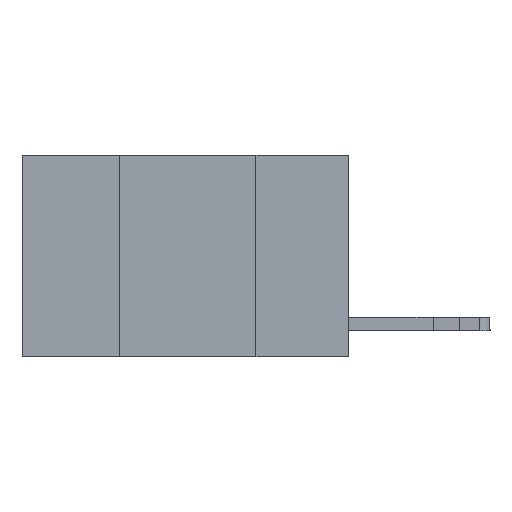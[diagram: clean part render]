
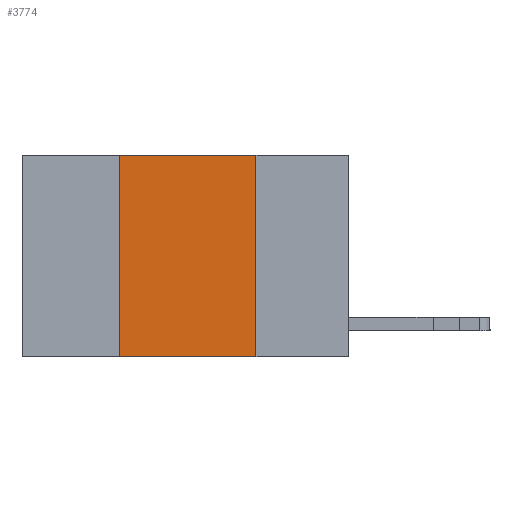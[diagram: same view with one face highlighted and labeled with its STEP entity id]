
A CAD part, left-side view. The second image highlights one B-rep face of the part: STEP entity #3774.
In plain terms, the highlighted planar face has unit normal (-1, 0, 0).
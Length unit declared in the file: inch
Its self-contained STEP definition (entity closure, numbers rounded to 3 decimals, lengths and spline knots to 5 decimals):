
#254 = EDGE_LOOP ( 'NONE', ( #4907, #4787, #3917, #13161 ) ) ;
#516 = LINE ( 'NONE', #7044, #6135 ) ;
#1281 = DIRECTION ( 'NONE',  ( 0., -1., 0. ) ) ;
#1306 = EDGE_CURVE ( 'NONE', #3032, #5021, #10308, .T. ) ;
#1442 = LINE ( 'NONE', #4758, #10505 ) ;
#1938 = AXIS2_PLACEMENT_3D ( 'NONE', #4579, #7053, #9041 ) ;
#2400 = LINE ( 'NONE', #3845, #10795 ) ;
#2567 = EDGE_CURVE ( 'NONE', #10927, #14480, #1442, .T. ) ;
#2594 = CARTESIAN_POINT ( 'NONE',  ( 0., 0.42, -0.37 ) ) ;
#2740 = DIRECTION ( 'NONE',  ( 0., -1., 0. ) ) ;
#3032 = VERTEX_POINT ( 'NONE', #6778 ) ;
#3354 = CARTESIAN_POINT ( 'NONE',  ( 0., 0.42, 0. ) ) ;
#3431 = DIRECTION ( 'NONE',  ( 0., 0., -1. ) ) ;
#3620 = PLANE ( 'NONE',  #1938 ) ;
#3629 = VECTOR ( 'NONE', #3431, 39.37008 ) ;
#3774 = ADVANCED_FACE ( 'NONE', ( #6984 ), #3620, .F. ) ;
#3845 = CARTESIAN_POINT ( 'NONE',  ( 0., 0.6, 0. ) ) ;
#3917 = ORIENTED_EDGE ( 'NONE', *, *, #2567, .F. ) ;
#4579 = CARTESIAN_POINT ( 'NONE',  ( 0., 0.6, 0. ) ) ;
#4758 = CARTESIAN_POINT ( 'NONE',  ( 0., 0.42, 0. ) ) ;
#4787 = ORIENTED_EDGE ( 'NONE', *, *, #10604, .F. ) ;
#4907 = ORIENTED_EDGE ( 'NONE', *, *, #1306, .F. ) ;
#5021 = VERTEX_POINT ( 'NONE', #13364 ) ;
#6135 = VECTOR ( 'NONE', #2740, 39.37008 ) ;
#6778 = CARTESIAN_POINT ( 'NONE',  ( 0., 0.17, 0. ) ) ;
#6984 = FACE_OUTER_BOUND ( 'NONE', #254, .T. ) ;
#7011 = CARTESIAN_POINT ( 'NONE',  ( 0., 0.17, 0. ) ) ;
#7044 = CARTESIAN_POINT ( 'NONE',  ( 0., 0.6, -0.37 ) ) ;
#7053 = DIRECTION ( 'NONE',  ( 1., 0., 0. ) ) ;
#9041 = DIRECTION ( 'NONE',  ( 0., 0., -1. ) ) ;
#9306 = EDGE_CURVE ( 'NONE', #10927, #5021, #516, .T. ) ;
#10308 = LINE ( 'NONE', #7011, #3629 ) ;
#10505 = VECTOR ( 'NONE', #11397, 39.37008 ) ;
#10604 = EDGE_CURVE ( 'NONE', #14480, #3032, #2400, .T. ) ;
#10795 = VECTOR ( 'NONE', #1281, 39.37008 ) ;
#10927 = VERTEX_POINT ( 'NONE', #2594 ) ;
#11397 = DIRECTION ( 'NONE',  ( 0., 0., 1. ) ) ;
#13161 = ORIENTED_EDGE ( 'NONE', *, *, #9306, .T. ) ;
#13364 = CARTESIAN_POINT ( 'NONE',  ( 0., 0.17, -0.37 ) ) ;
#14480 = VERTEX_POINT ( 'NONE', #3354 ) ;
